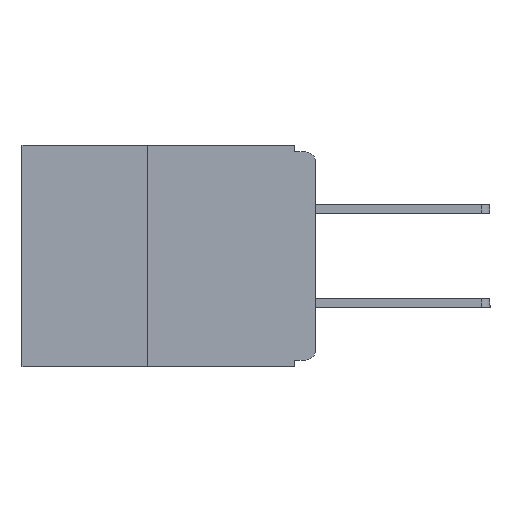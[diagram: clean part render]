
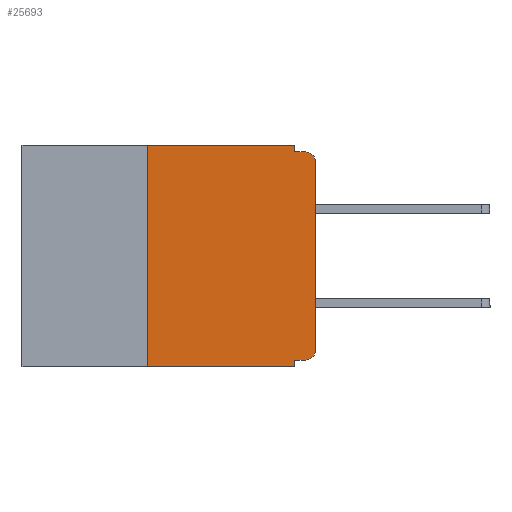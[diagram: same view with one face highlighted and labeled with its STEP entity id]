
A CAD part, left-side view. The second image highlights one B-rep face of the part: STEP entity #25693.
In plain terms, the highlighted planar face has unit normal (-1, 0, 0).
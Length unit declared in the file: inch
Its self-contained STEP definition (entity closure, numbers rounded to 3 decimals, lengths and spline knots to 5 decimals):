
#628 = ORIENTED_EDGE ( 'NONE', *, *, #10531, .T. ) ;
#762 = VECTOR ( 'NONE', #32979, 39.37008 ) ;
#776 = ORIENTED_EDGE ( 'NONE', *, *, #28559, .F. ) ;
#1553 = EDGE_LOOP ( 'NONE', ( #628, #17472, #11634, #14042, #776, #10833, #2261, #29482, #28401, #15339 ) ) ;
#1682 = PLANE ( 'NONE',  #22606 ) ;
#1741 = FACE_OUTER_BOUND ( 'NONE', #1553, .T. ) ;
#1850 = CARTESIAN_POINT ( 'NONE',  ( 0., 0., -0.025 ) ) ;
#2090 = CARTESIAN_POINT ( 'NONE',  ( 0., 0.031, -0.32 ) ) ;
#2235 = VECTOR ( 'NONE', #30560, 39.37008 ) ;
#2261 = ORIENTED_EDGE ( 'NONE', *, *, #26477, .T. ) ;
#3782 = CARTESIAN_POINT ( 'NONE',  ( 0., 0.015, -0.025 ) ) ;
#4424 = VERTEX_POINT ( 'NONE', #20876 ) ;
#4562 = DIRECTION ( 'NONE',  ( 0., 0., -1. ) ) ;
#5259 = VECTOR ( 'NONE', #35355, 39.37008 ) ;
#5599 = LINE ( 'NONE', #24574, #34122 ) ;
#6125 = CARTESIAN_POINT ( 'NONE',  ( 0., 0.031, -0.33 ) ) ;
#6479 = VERTEX_POINT ( 'NONE', #7819 ) ;
#6656 = DIRECTION ( 'NONE',  ( 0., 0., -1. ) ) ;
#6784 = EDGE_CURVE ( 'NONE', #20432, #4424, #28900, .T. ) ;
#7805 = DIRECTION ( 'NONE',  ( 0., -1., 0. ) ) ;
#7808 = LINE ( 'NONE', #26025, #21882 ) ;
#7819 = CARTESIAN_POINT ( 'NONE',  ( 0., 0.015, -0.01 ) ) ;
#8534 = CARTESIAN_POINT ( 'NONE',  ( 0., 0., -0.01 ) ) ;
#8536 = VERTEX_POINT ( 'NONE', #25283 ) ;
#9270 = CARTESIAN_POINT ( 'NONE',  ( 0., 0.015, -0.32 ) ) ;
#9843 = EDGE_CURVE ( 'NONE', #16483, #6479, #35282, .T. ) ;
#10531 = EDGE_CURVE ( 'NONE', #4424, #16483, #18879, .T. ) ;
#10833 = ORIENTED_EDGE ( 'NONE', *, *, #11130, .F. ) ;
#11100 = LINE ( 'NONE', #27364, #5259 ) ;
#11130 = EDGE_CURVE ( 'NONE', #17511, #18790, #7808, .T. ) ;
#11634 = ORIENTED_EDGE ( 'NONE', *, *, #21171, .F. ) ;
#11854 = LINE ( 'NONE', #34456, #18444 ) ;
#14042 = ORIENTED_EDGE ( 'NONE', *, *, #27762, .F. ) ;
#15339 = ORIENTED_EDGE ( 'NONE', *, *, #6784, .T. ) ;
#15613 = DIRECTION ( 'NONE',  ( -1., 0., 0. ) ) ;
#15756 = CARTESIAN_POINT ( 'NONE',  ( 0., 0.437, 0. ) ) ;
#16199 = VECTOR ( 'NONE', #17165, 39.37008 ) ;
#16483 = VERTEX_POINT ( 'NONE', #1850 ) ;
#17147 = VERTEX_POINT ( 'NONE', #21835 ) ;
#17165 = DIRECTION ( 'NONE',  ( 0., 1., 0. ) ) ;
#17472 = ORIENTED_EDGE ( 'NONE', *, *, #9843, .T. ) ;
#17511 = VERTEX_POINT ( 'NONE', #20721 ) ;
#18218 = CARTESIAN_POINT ( 'NONE',  ( 0., 0.25, 0. ) ) ;
#18444 = VECTOR ( 'NONE', #21026, 39.37008 ) ;
#18790 = VERTEX_POINT ( 'NONE', #18218 ) ;
#18879 = LINE ( 'NONE', #26301, #25339 ) ;
#20270 = AXIS2_PLACEMENT_3D ( 'NONE', #3782, #23499, #6656 ) ;
#20432 = VERTEX_POINT ( 'NONE', #9270 ) ;
#20721 = CARTESIAN_POINT ( 'NONE',  ( 0., 0.25, -0.33 ) ) ;
#20876 = CARTESIAN_POINT ( 'NONE',  ( 0., 0., -0.305 ) ) ;
#21026 = DIRECTION ( 'NONE',  ( 0., 0., -1. ) ) ;
#21171 = EDGE_CURVE ( 'NONE', #17147, #6479, #22991, .T. ) ;
#21473 = DIRECTION ( 'NONE',  ( 1., 0., 0. ) ) ;
#21632 = VERTEX_POINT ( 'NONE', #2090 ) ;
#21835 = CARTESIAN_POINT ( 'NONE',  ( 0., 0.031, -0.01 ) ) ;
#21882 = VECTOR ( 'NONE', #28755, 39.37008 ) ;
#22606 = AXIS2_PLACEMENT_3D ( 'NONE', #15756, #21473, #4562 ) ;
#22991 = LINE ( 'NONE', #8534, #2235 ) ;
#23019 = EDGE_CURVE ( 'NONE', #20432, #21632, #23580, .T. ) ;
#23092 = VERTEX_POINT ( 'NONE', #6125 ) ;
#23499 = DIRECTION ( 'NONE',  ( -1., 0., 0. ) ) ;
#23580 = LINE ( 'NONE', #33467, #16199 ) ;
#24574 = CARTESIAN_POINT ( 'NONE',  ( 0., 0.437, 0. ) ) ;
#25283 = CARTESIAN_POINT ( 'NONE',  ( 0., 0.031, 0. ) ) ;
#25339 = VECTOR ( 'NONE', #28912, 39.37008 ) ;
#25513 = AXIS2_PLACEMENT_3D ( 'NONE', #32010, #15613, #34628 ) ;
#25693 = ADVANCED_FACE ( 'NONE', ( #1741 ), #1682, .F. ) ;
#26025 = CARTESIAN_POINT ( 'NONE',  ( 0., 0.25, -0.33 ) ) ;
#26301 = CARTESIAN_POINT ( 'NONE',  ( 0., 0., 0. ) ) ;
#26477 = EDGE_CURVE ( 'NONE', #17511, #23092, #11100, .T. ) ;
#26528 = EDGE_CURVE ( 'NONE', #21632, #23092, #29677, .T. ) ;
#27364 = CARTESIAN_POINT ( 'NONE',  ( 0., 0.437, -0.33 ) ) ;
#27591 = CARTESIAN_POINT ( 'NONE',  ( 0., 0.031, -0.33 ) ) ;
#27762 = EDGE_CURVE ( 'NONE', #8536, #17147, #11854, .T. ) ;
#28401 = ORIENTED_EDGE ( 'NONE', *, *, #23019, .F. ) ;
#28559 = EDGE_CURVE ( 'NONE', #18790, #8536, #5599, .T. ) ;
#28755 = DIRECTION ( 'NONE',  ( 0., 0., 1. ) ) ;
#28900 = CIRCLE ( 'NONE', #25513, 0.015 ) ;
#28912 = DIRECTION ( 'NONE',  ( 0., 0., 1. ) ) ;
#29482 = ORIENTED_EDGE ( 'NONE', *, *, #26528, .F. ) ;
#29677 = LINE ( 'NONE', #27591, #762 ) ;
#30560 = DIRECTION ( 'NONE',  ( 0., -1., 0. ) ) ;
#32010 = CARTESIAN_POINT ( 'NONE',  ( 0., 0.015, -0.305 ) ) ;
#32979 = DIRECTION ( 'NONE',  ( 0., 0., -1. ) ) ;
#33467 = CARTESIAN_POINT ( 'NONE',  ( 0., 0., -0.32 ) ) ;
#34122 = VECTOR ( 'NONE', #7805, 39.37008 ) ;
#34456 = CARTESIAN_POINT ( 'NONE',  ( 0., 0.031, 0. ) ) ;
#34628 = DIRECTION ( 'NONE',  ( 0., 0., -1. ) ) ;
#35282 = CIRCLE ( 'NONE', #20270, 0.015 ) ;
#35355 = DIRECTION ( 'NONE',  ( 0., -1., 0. ) ) ;
